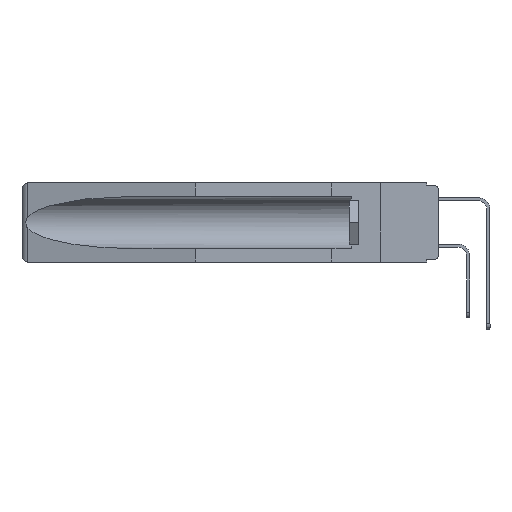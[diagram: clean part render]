
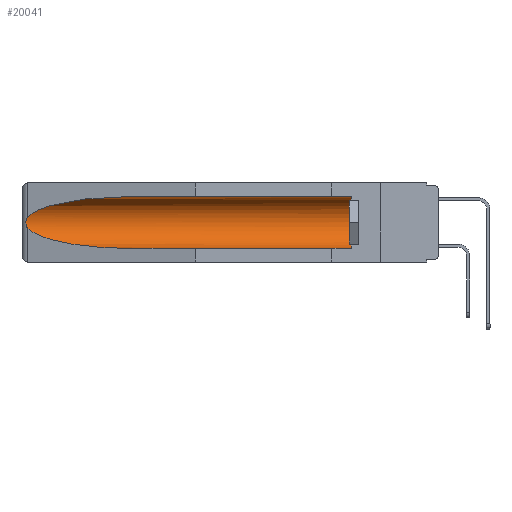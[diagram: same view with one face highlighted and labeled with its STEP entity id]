
A CAD part, left-side view. The second image highlights one B-rep face of the part: STEP entity #20041.
In plain terms, the highlighted cylindrical face has radius 2.857 mm (diameter 5.715 mm), a partial arc.
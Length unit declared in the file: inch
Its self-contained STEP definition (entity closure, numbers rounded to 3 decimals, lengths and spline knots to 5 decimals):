
#113 = VECTOR ( 'NONE', #2034, 39.37008 ) ;
#140 = CARTESIAN_POINT ( 'NONE',  ( 0.26537, 1.52718, -0.14972 ) ) ;
#240 = DIRECTION ( 'NONE',  ( 0., 0., 1. ) ) ;
#245 = CARTESIAN_POINT ( 'NONE',  ( 0.155, -0.30754, -0.059 ) ) ;
#294 = ORIENTED_EDGE ( 'NONE', *, *, #18865, .T. ) ;
#587 = EDGE_CURVE ( 'NONE', #13516, #7918, #21232, .T. ) ;
#820 = CARTESIAN_POINT ( 'NONE',  ( 0.26537, 1.52718, -0.19328 ) ) ;
#995 = AXIS2_PLACEMENT_3D ( 'NONE', #17858, #7870, #12804 ) ;
#1548 = DIRECTION ( 'NONE',  ( 0., 1., 0. ) ) ;
#1857 = CARTESIAN_POINT ( 'NONE',  ( 0.26597, 1.52961, -0.15275 ) ) ;
#1918 = EDGE_CURVE ( 'NONE', #7918, #5760, #17377, .T. ) ;
#2034 = DIRECTION ( 'NONE',  ( 0., 1., 0. ) ) ;
#2575 =( BOUNDED_CURVE ( )  B_SPLINE_CURVE ( 3, ( #10252, #6692, #8575, #15432 ),
 .UNSPECIFIED., .F., .F. ) 
 B_SPLINE_CURVE_WITH_KNOTS ( ( 4, 4 ),
 ( 0.1948, 1.5708 ),
 .UNSPECIFIED. ) 
 CURVE ( )  GEOMETRIC_REPRESENTATION_ITEM ( )  RATIONAL_B_SPLINE_CURVE ( ( 1., 0.848, 0.848, 1. ) ) 
 REPRESENTATION_ITEM ( '' )  );
#2788 = B_SPLINE_CURVE_WITH_KNOTS ( 'NONE', 3,
 ( #17409, #1857, #7310, #8996, #8661, #13945, #6985, #10889, #5645, #15957 ),
 .UNSPECIFIED., .F., .F.,
 ( 4, 2, 2, 2, 4 ),
 ( 0., 0.00029, 0.00058, 0.00087, 0.00117 ),
 .UNSPECIFIED. ) ;
#2923 = ORIENTED_EDGE ( 'NONE', *, *, #1918, .T. ) ;
#3703 = DIRECTION ( 'NONE',  ( 0., -1., 0. ) ) ;
#3834 = CARTESIAN_POINT ( 'NONE',  ( 0.155, 1.07973, -0.059 ) ) ;
#4700 = ORIENTED_EDGE ( 'NONE', *, *, #587, .T. ) ;
#5645 = CARTESIAN_POINT ( 'NONE',  ( 0.26597, 1.5296, -0.19026 ) ) ;
#5760 = VERTEX_POINT ( 'NONE', #19667 ) ;
#5783 = EDGE_LOOP ( 'NONE', ( #20209, #16267, #294, #18178, #4700, #2923 ) ) ;
#6692 = CARTESIAN_POINT ( 'NONE',  ( 0.25451, 1.48313, -0.24835 ) ) ;
#6985 = CARTESIAN_POINT ( 'NONE',  ( 0.2673, 1.53269, -0.17917 ) ) ;
#7310 = CARTESIAN_POINT ( 'NONE',  ( 0.26654, 1.53092, -0.15636 ) ) ;
#7624 = AXIS2_PLACEMENT_3D ( 'NONE', #14029, #3703, #240 ) ;
#7870 = DIRECTION ( 'NONE',  ( 0., 1., 0. ) ) ;
#7918 = VERTEX_POINT ( 'NONE', #17730 ) ;
#7926 = VERTEX_POINT ( 'NONE', #820 ) ;
#8210 = VERTEX_POINT ( 'NONE', #20622 ) ;
#8575 = CARTESIAN_POINT ( 'NONE',  ( 0.21114, 1.30732, -0.284 ) ) ;
#8661 = CARTESIAN_POINT ( 'NONE',  ( 0.2675, 1.53308, -0.16763 ) ) ;
#8996 = CARTESIAN_POINT ( 'NONE',  ( 0.2673, 1.5327, -0.16383 ) ) ;
#9072 = CARTESIAN_POINT ( 'NONE',  ( 0.26537, 1.52718, -0.14972 ) ) ;
#10095 = CARTESIAN_POINT ( 'NONE',  ( 0.155, 0.126, -0.284 ) ) ;
#10252 = CARTESIAN_POINT ( 'NONE',  ( 0.26537, 1.52718, -0.19328 ) ) ;
#10812 =( BOUNDED_CURVE ( )  B_SPLINE_CURVE ( 3, ( #3834, #15491, #17383, #9072 ),
 .UNSPECIFIED., .F., .T. ) 
 B_SPLINE_CURVE_WITH_KNOTS ( ( 4, 4 ),
 ( 4.71239, 6.08839 ),
 .UNSPECIFIED. ) 
 CURVE ( )  GEOMETRIC_REPRESENTATION_ITEM ( )  RATIONAL_B_SPLINE_CURVE ( ( 1., 0.848, 0.848, 1. ) ) 
 REPRESENTATION_ITEM ( '' )  );
#10889 = CARTESIAN_POINT ( 'NONE',  ( 0.26655, 1.53094, -0.18657 ) ) ;
#11335 = FACE_OUTER_BOUND ( 'NONE', #5783, .T. ) ;
#11833 = CARTESIAN_POINT ( 'NONE',  ( 0.155, -0.30754, -0.284 ) ) ;
#12134 = VERTEX_POINT ( 'NONE', #140 ) ;
#12691 = CYLINDRICAL_SURFACE ( 'NONE', #995, 0.1125 ) ;
#12804 = DIRECTION ( 'NONE',  ( 0., 0., 1. ) ) ;
#13516 = VERTEX_POINT ( 'NONE', #10095 ) ;
#13945 = CARTESIAN_POINT ( 'NONE',  ( 0.2675, 1.53308, -0.17534 ) ) ;
#14029 = CARTESIAN_POINT ( 'NONE',  ( 0.155, 0.126, -0.1715 ) ) ;
#15432 = CARTESIAN_POINT ( 'NONE',  ( 0.155, 1.07973, -0.284 ) ) ;
#15491 = CARTESIAN_POINT ( 'NONE',  ( 0.21114, 1.30732, -0.059 ) ) ;
#15957 = CARTESIAN_POINT ( 'NONE',  ( 0.26537, 1.52718, -0.19328 ) ) ;
#16267 = ORIENTED_EDGE ( 'NONE', *, *, #19903, .T. ) ;
#16367 = VECTOR ( 'NONE', #1548, 39.37008 ) ;
#17377 = LINE ( 'NONE', #245, #113 ) ;
#17383 = CARTESIAN_POINT ( 'NONE',  ( 0.25451, 1.48313, -0.09465 ) ) ;
#17409 = CARTESIAN_POINT ( 'NONE',  ( 0.26537, 1.52718, -0.14972 ) ) ;
#17730 = CARTESIAN_POINT ( 'NONE',  ( 0.155, 0.126, -0.059 ) ) ;
#17858 = CARTESIAN_POINT ( 'NONE',  ( 0.155, -0.30754, -0.1715 ) ) ;
#18178 = ORIENTED_EDGE ( 'NONE', *, *, #19830, .F. ) ;
#18865 = EDGE_CURVE ( 'NONE', #7926, #8210, #2575, .T. ) ;
#19667 = CARTESIAN_POINT ( 'NONE',  ( 0.155, 1.07973, -0.059 ) ) ;
#19830 = EDGE_CURVE ( 'NONE', #13516, #8210, #20358, .T. ) ;
#19903 = EDGE_CURVE ( 'NONE', #12134, #7926, #2788, .T. ) ;
#20041 = ADVANCED_FACE ( 'NONE', ( #11335 ), #12691, .F. ) ;
#20209 = ORIENTED_EDGE ( 'NONE', *, *, #20325, .T. ) ;
#20325 = EDGE_CURVE ( 'NONE', #5760, #12134, #10812, .T. ) ;
#20358 = LINE ( 'NONE', #11833, #16367 ) ;
#20622 = CARTESIAN_POINT ( 'NONE',  ( 0.155, 1.07973, -0.284 ) ) ;
#21232 = CIRCLE ( 'NONE', #7624, 0.1125 ) ;
